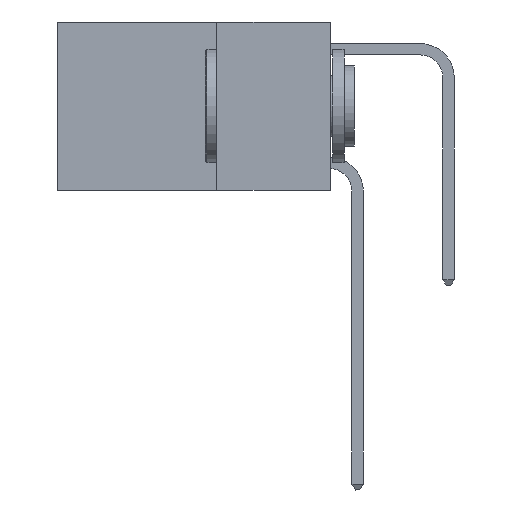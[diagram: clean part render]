
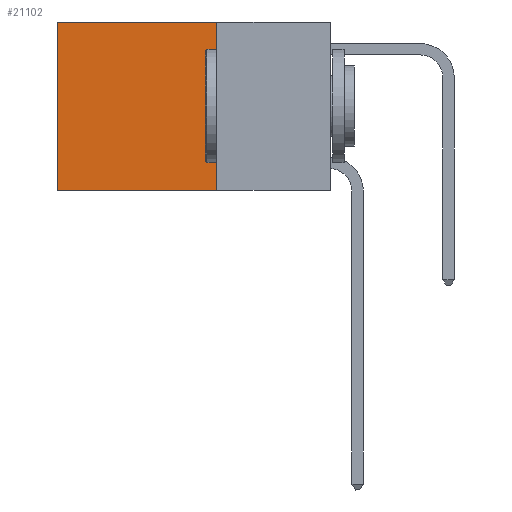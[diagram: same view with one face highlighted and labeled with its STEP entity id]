
A CAD part, left-side view. The second image highlights one B-rep face of the part: STEP entity #21102.
In plain terms, the highlighted planar face has unit normal (-1, 0, 0).
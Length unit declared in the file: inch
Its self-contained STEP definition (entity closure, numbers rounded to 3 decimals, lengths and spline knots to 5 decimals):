
#48 = EDGE_CURVE ( 'NONE', #8300, #20899, #1895, .T. ) ;
#183 = ORIENTED_EDGE ( 'NONE', *, *, #48, .T. ) ;
#1835 = CARTESIAN_POINT ( 'NONE',  ( 0.2625, 0.6, 0. ) ) ;
#1895 = LINE ( 'NONE', #16244, #5904 ) ;
#1908 = LINE ( 'NONE', #5253, #18433 ) ;
#3794 = DIRECTION ( 'NONE',  ( 0., 0., -1. ) ) ;
#3872 = EDGE_LOOP ( 'NONE', ( #183, #18683, #13931, #19143 ) ) ;
#4103 = EDGE_CURVE ( 'NONE', #17149, #12597, #5874, .T. ) ;
#4371 = DIRECTION ( 'NONE',  ( 0., 1., 0. ) ) ;
#4486 = CARTESIAN_POINT ( 'NONE',  ( 0.2625, 0.25, 0. ) ) ;
#5253 = CARTESIAN_POINT ( 'NONE',  ( 0.2625, 0.25, -0.37 ) ) ;
#5874 = LINE ( 'NONE', #10801, #7152 ) ;
#5904 = VECTOR ( 'NONE', #3794, 39.37008 ) ;
#5954 = FACE_OUTER_BOUND ( 'NONE', #3872, .T. ) ;
#7010 = CARTESIAN_POINT ( 'NONE',  ( 0.2625, 0.25, -0.37 ) ) ;
#7152 = VECTOR ( 'NONE', #18166, 39.37008 ) ;
#8300 = VERTEX_POINT ( 'NONE', #1835 ) ;
#9685 = EDGE_CURVE ( 'NONE', #17149, #8300, #15497, .T. ) ;
#10307 = EDGE_CURVE ( 'NONE', #12597, #20899, #1908, .T. ) ;
#10801 = CARTESIAN_POINT ( 'NONE',  ( 0.2625, 0.25, 0. ) ) ;
#12597 = VERTEX_POINT ( 'NONE', #7010 ) ;
#13252 = CARTESIAN_POINT ( 'NONE',  ( 0.2625, 0.25, 0. ) ) ;
#13931 = ORIENTED_EDGE ( 'NONE', *, *, #4103, .F. ) ;
#14573 = DIRECTION ( 'NONE',  ( 0., 1., 0. ) ) ;
#15497 = LINE ( 'NONE', #4486, #19157 ) ;
#16244 = CARTESIAN_POINT ( 'NONE',  ( 0.2625, 0.6, 0. ) ) ;
#16347 = CARTESIAN_POINT ( 'NONE',  ( 0.2625, 0.6, -0.37 ) ) ;
#16938 = PLANE ( 'NONE',  #19101 ) ;
#17149 = VERTEX_POINT ( 'NONE', #18284 ) ;
#18166 = DIRECTION ( 'NONE',  ( 0., 0., -1. ) ) ;
#18284 = CARTESIAN_POINT ( 'NONE',  ( 0.2625, 0.25, 0. ) ) ;
#18433 = VECTOR ( 'NONE', #14573, 39.37008 ) ;
#18683 = ORIENTED_EDGE ( 'NONE', *, *, #10307, .F. ) ;
#19101 = AXIS2_PLACEMENT_3D ( 'NONE', #13252, #20123, #20480 ) ;
#19143 = ORIENTED_EDGE ( 'NONE', *, *, #9685, .T. ) ;
#19157 = VECTOR ( 'NONE', #4371, 39.37008 ) ;
#20123 = DIRECTION ( 'NONE',  ( 1., 0., 0. ) ) ;
#20480 = DIRECTION ( 'NONE',  ( 0., 0., -1. ) ) ;
#20899 = VERTEX_POINT ( 'NONE', #16347 ) ;
#21102 = ADVANCED_FACE ( 'NONE', ( #5954 ), #16938, .F. ) ;
